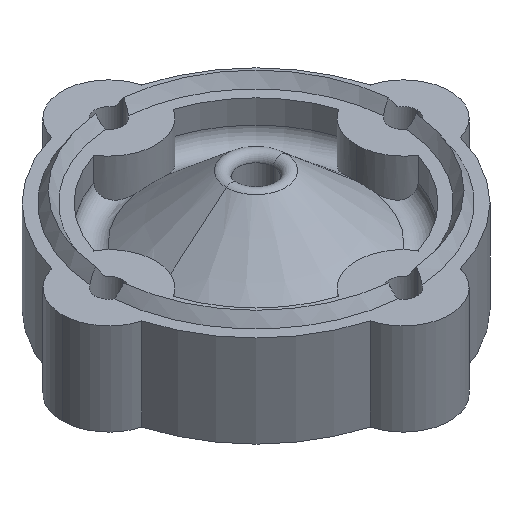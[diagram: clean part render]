
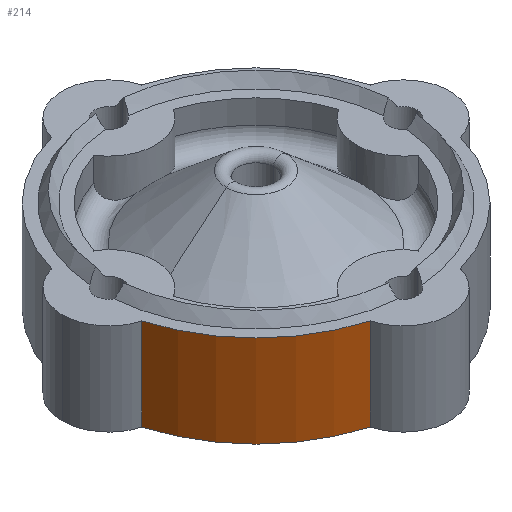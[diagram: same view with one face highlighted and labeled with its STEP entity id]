
A CAD part, isometric view. The second image highlights one B-rep face of the part: STEP entity #214.
In plain terms, the highlighted cylindrical face has radius 45 mm (diameter 90 mm), a partial arc.
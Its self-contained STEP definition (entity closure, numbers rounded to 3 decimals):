
#86 = EDGE_CURVE ( 'NONE', #1427, #1461, #1512, .T. ) ;
#152 = VECTOR ( 'NONE', #1188, 1000. ) ;
#186 = DIRECTION ( 'NONE',  ( 0., 0., 1. ) ) ;
#214 = ADVANCED_FACE ( 'NONE', ( #269 ), #1629, .T. ) ;
#269 = FACE_OUTER_BOUND ( 'NONE', #1867, .T. ) ;
#382 = CARTESIAN_POINT ( 'NONE',  ( -12.265, -43.296, 0. ) ) ;
#415 = AXIS2_PLACEMENT_3D ( 'NONE', #1524, #186, #1102 ) ;
#477 = CARTESIAN_POINT ( 'NONE',  ( -12.265, -43.296, -25. ) ) ;
#594 = CIRCLE ( 'NONE', #1275, 45. ) ;
#617 = ORIENTED_EDGE ( 'NONE', *, *, #1092, .T. ) ;
#730 = CARTESIAN_POINT ( 'NONE',  ( 0., 0., 0. ) ) ;
#835 = CARTESIAN_POINT ( 'NONE',  ( -43.296, -12.265, 0. ) ) ;
#949 = DIRECTION ( 'NONE',  ( 0., 0., -1. ) ) ;
#997 = EDGE_CURVE ( 'NONE', #1112, #1461, #1790, .T. ) ;
#1011 = ORIENTED_EDGE ( 'NONE', *, *, #1870, .T. ) ;
#1092 = EDGE_CURVE ( 'NONE', #1931, #1112, #594, .T. ) ;
#1097 = CARTESIAN_POINT ( 'NONE',  ( -43.296, -12.265, -25. ) ) ;
#1102 = DIRECTION ( 'NONE',  ( 1., 0., 0. ) ) ;
#1112 = VERTEX_POINT ( 'NONE', #477 ) ;
#1166 = DIRECTION ( 'NONE',  ( 0., 0., 1. ) ) ;
#1188 = DIRECTION ( 'NONE',  ( 0., 0., 1. ) ) ;
#1275 = AXIS2_PLACEMENT_3D ( 'NONE', #1493, #1525, #1825 ) ;
#1325 = DIRECTION ( 'NONE',  ( 1., 0., 0. ) ) ;
#1406 = LINE ( 'NONE', #1526, #1429 ) ;
#1427 = VERTEX_POINT ( 'NONE', #835 ) ;
#1429 = VECTOR ( 'NONE', #949, 1000. ) ;
#1461 = VERTEX_POINT ( 'NONE', #382 ) ;
#1493 = CARTESIAN_POINT ( 'NONE',  ( 0., 0., -25. ) ) ;
#1512 = CIRCLE ( 'NONE', #415, 45. ) ;
#1524 = CARTESIAN_POINT ( 'NONE',  ( 0., 0., 0. ) ) ;
#1525 = DIRECTION ( 'NONE',  ( 0., 0., 1. ) ) ;
#1526 = CARTESIAN_POINT ( 'NONE',  ( -43.296, -12.265, -12.5 ) ) ;
#1629 = CYLINDRICAL_SURFACE ( 'NONE', #1860, 45. ) ;
#1701 = ORIENTED_EDGE ( 'NONE', *, *, #997, .T. ) ;
#1790 = LINE ( 'NONE', #1900, #152 ) ;
#1825 = DIRECTION ( 'NONE',  ( 1., 0., 0. ) ) ;
#1860 = AXIS2_PLACEMENT_3D ( 'NONE', #730, #1166, #1325 ) ;
#1867 = EDGE_LOOP ( 'NONE', ( #617, #1701, #1888, #1011 ) ) ;
#1870 = EDGE_CURVE ( 'NONE', #1427, #1931, #1406, .T. ) ;
#1888 = ORIENTED_EDGE ( 'NONE', *, *, #86, .F. ) ;
#1900 = CARTESIAN_POINT ( 'NONE',  ( -12.265, -43.296, -12.5 ) ) ;
#1931 = VERTEX_POINT ( 'NONE', #1097 ) ;
